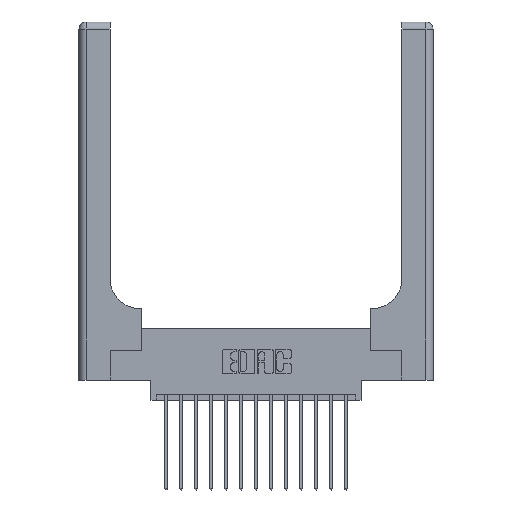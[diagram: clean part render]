
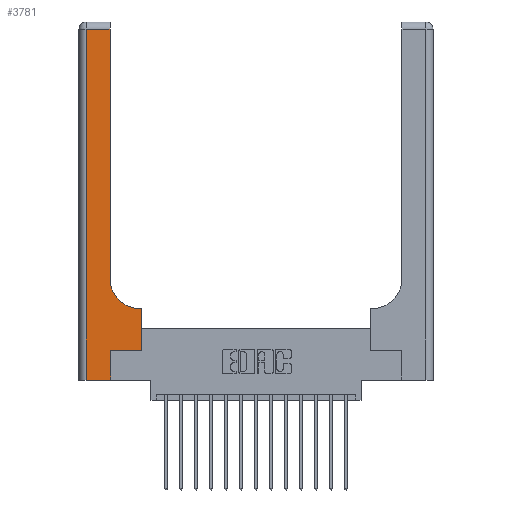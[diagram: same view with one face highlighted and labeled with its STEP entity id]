
A CAD part, top view. The second image highlights one B-rep face of the part: STEP entity #3781.
In plain terms, the highlighted planar face has unit normal (0, 0, 1).
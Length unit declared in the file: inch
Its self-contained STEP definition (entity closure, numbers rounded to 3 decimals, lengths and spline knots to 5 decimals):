
#45 = VECTOR ( 'NONE', #6647, 39.37008 ) ;
#203 = LINE ( 'NONE', #4536, #538 ) ;
#216 = VERTEX_POINT ( 'NONE', #15175 ) ;
#538 = VECTOR ( 'NONE', #15731, 39.37008 ) ;
#841 = EDGE_LOOP ( 'NONE', ( #7675, #12530, #7715, #9164, #15909, #1863, #8410, #17644, #9379 ) ) ;
#1042 = LINE ( 'NONE', #16541, #10426 ) ;
#1676 = CARTESIAN_POINT ( 'NONE',  ( 0.26, 0.6, 0.37 ) ) ;
#1863 = ORIENTED_EDGE ( 'NONE', *, *, #10419, .T. ) ;
#2457 = DIRECTION ( 'NONE',  ( 1., 0., 0. ) ) ;
#2680 = LINE ( 'NONE', #18099, #11382 ) ;
#3426 = AXIS2_PLACEMENT_3D ( 'NONE', #14814, #9149, #10886 ) ;
#3527 = LINE ( 'NONE', #14712, #7676 ) ;
#3568 = VERTEX_POINT ( 'NONE', #17284 ) ;
#3571 = DIRECTION ( 'NONE',  ( 0., 0., -1. ) ) ;
#3777 = EDGE_CURVE ( 'NONE', #4662, #13341, #5003, .T. ) ;
#3781 = ADVANCED_FACE ( 'NONE', ( #10627 ), #17745, .F. ) ;
#4006 = DIRECTION ( 'NONE',  ( 0., 1., 0. ) ) ;
#4119 = CIRCLE ( 'NONE', #6470, 0.25 ) ;
#4270 = CARTESIAN_POINT ( 'NONE',  ( 0.265, 0., 0.37 ) ) ;
#4536 = CARTESIAN_POINT ( 'NONE',  ( 0.528, 0.25, 0.37 ) ) ;
#4662 = VERTEX_POINT ( 'NONE', #15918 ) ;
#5003 = LINE ( 'NONE', #15000, #12500 ) ;
#5441 = CARTESIAN_POINT ( 'NONE',  ( 0.06, 3., 0.37 ) ) ;
#5740 = VERTEX_POINT ( 'NONE', #14262 ) ;
#5836 = EDGE_CURVE ( 'NONE', #13341, #17510, #13593, .T. ) ;
#6186 = EDGE_CURVE ( 'NONE', #6664, #16055, #2680, .T. ) ;
#6470 = AXIS2_PLACEMENT_3D ( 'NONE', #16122, #3571, #2457 ) ;
#6647 = DIRECTION ( 'NONE',  ( 0., -1., 0. ) ) ;
#6664 = VERTEX_POINT ( 'NONE', #4270 ) ;
#7200 = EDGE_CURVE ( 'NONE', #3568, #216, #4119, .T. ) ;
#7675 = ORIENTED_EDGE ( 'NONE', *, *, #12628, .T. ) ;
#7676 = VECTOR ( 'NONE', #13327, 39.37008 ) ;
#7715 = ORIENTED_EDGE ( 'NONE', *, *, #5836, .T. ) ;
#8410 = ORIENTED_EDGE ( 'NONE', *, *, #9157, .T. ) ;
#8948 = VECTOR ( 'NONE', #15145, 39.37008 ) ;
#9149 = DIRECTION ( 'NONE',  ( 0., 0., -1. ) ) ;
#9157 = EDGE_CURVE ( 'NONE', #5740, #16231, #203, .T. ) ;
#9164 = ORIENTED_EDGE ( 'NONE', *, *, #17938, .T. ) ;
#9379 = ORIENTED_EDGE ( 'NONE', *, *, #7200, .T. ) ;
#9974 = DIRECTION ( 'NONE',  ( 0., 1., 0. ) ) ;
#10270 = LINE ( 'NONE', #1676, #17908 ) ;
#10419 = EDGE_CURVE ( 'NONE', #16055, #5740, #3527, .T. ) ;
#10426 = VECTOR ( 'NONE', #4006, 39.37008 ) ;
#10627 = FACE_OUTER_BOUND ( 'NONE', #841, .T. ) ;
#10769 = CARTESIAN_POINT ( 'NONE',  ( 0.528, 0.6, 0.37 ) ) ;
#10886 = DIRECTION ( 'NONE',  ( -1., 0., 0. ) ) ;
#10931 = LINE ( 'NONE', #16477, #8948 ) ;
#10949 = CARTESIAN_POINT ( 'NONE',  ( 0.06, 2.94, 0.37 ) ) ;
#11382 = VECTOR ( 'NONE', #9974, 39.37008 ) ;
#11525 = DIRECTION ( 'NONE',  ( -1., 0., 0. ) ) ;
#12141 = DIRECTION ( 'NONE',  ( -1., 0., 0. ) ) ;
#12500 = VECTOR ( 'NONE', #12141, 39.37008 ) ;
#12530 = ORIENTED_EDGE ( 'NONE', *, *, #3777, .T. ) ;
#12628 = EDGE_CURVE ( 'NONE', #216, #4662, #1042, .T. ) ;
#12703 = EDGE_CURVE ( 'NONE', #16231, #3568, #10270, .T. ) ;
#13327 = DIRECTION ( 'NONE',  ( 1., 0., 0. ) ) ;
#13341 = VERTEX_POINT ( 'NONE', #10949 ) ;
#13577 = CARTESIAN_POINT ( 'NONE',  ( 0.06, 0., 0.37 ) ) ;
#13593 = LINE ( 'NONE', #5441, #45 ) ;
#14262 = CARTESIAN_POINT ( 'NONE',  ( 0.528, 0.25, 0.37 ) ) ;
#14712 = CARTESIAN_POINT ( 'NONE',  ( 0.265, 0.25, 0.37 ) ) ;
#14814 = CARTESIAN_POINT ( 'NONE',  ( 0., 3., 0.37 ) ) ;
#15000 = CARTESIAN_POINT ( 'NONE',  ( 0., 2.94, 0.37 ) ) ;
#15145 = DIRECTION ( 'NONE',  ( 1., 0., 0. ) ) ;
#15175 = CARTESIAN_POINT ( 'NONE',  ( 0.26, 0.85, 0.37 ) ) ;
#15731 = DIRECTION ( 'NONE',  ( 0., 1., 0. ) ) ;
#15802 = CARTESIAN_POINT ( 'NONE',  ( 0.265, 0.25, 0.37 ) ) ;
#15909 = ORIENTED_EDGE ( 'NONE', *, *, #6186, .T. ) ;
#15918 = CARTESIAN_POINT ( 'NONE',  ( 0.26, 2.94, 0.37 ) ) ;
#16055 = VERTEX_POINT ( 'NONE', #15802 ) ;
#16122 = CARTESIAN_POINT ( 'NONE',  ( 0.51, 0.85, 0.37 ) ) ;
#16231 = VERTEX_POINT ( 'NONE', #10769 ) ;
#16477 = CARTESIAN_POINT ( 'NONE',  ( 0., 0., 0.37 ) ) ;
#16541 = CARTESIAN_POINT ( 'NONE',  ( 0.26, 3., 0.37 ) ) ;
#17284 = CARTESIAN_POINT ( 'NONE',  ( 0.51, 0.6, 0.37 ) ) ;
#17510 = VERTEX_POINT ( 'NONE', #13577 ) ;
#17644 = ORIENTED_EDGE ( 'NONE', *, *, #12703, .T. ) ;
#17745 = PLANE ( 'NONE',  #3426 ) ;
#17908 = VECTOR ( 'NONE', #11525, 39.37008 ) ;
#17938 = EDGE_CURVE ( 'NONE', #17510, #6664, #10931, .T. ) ;
#18099 = CARTESIAN_POINT ( 'NONE',  ( 0.265, 0., 0.37 ) ) ;
